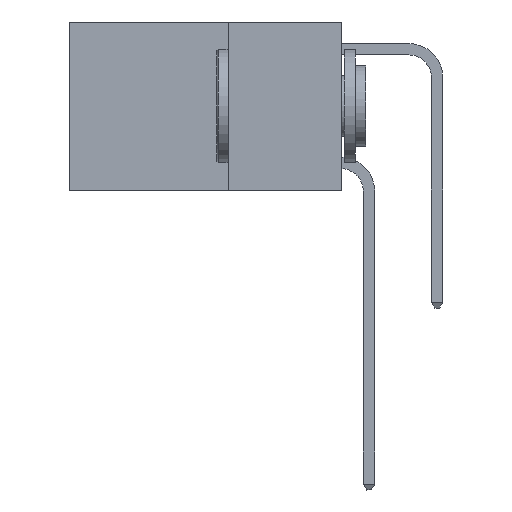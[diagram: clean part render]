
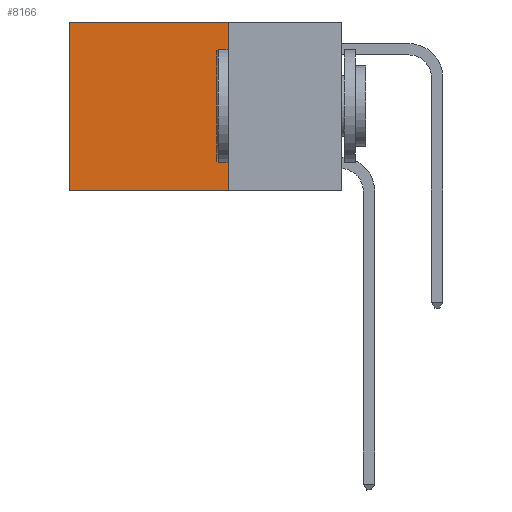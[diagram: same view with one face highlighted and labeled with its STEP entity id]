
A CAD part, left-side view. The second image highlights one B-rep face of the part: STEP entity #8166.
In plain terms, the highlighted planar face has unit normal (-1, 0, 0).
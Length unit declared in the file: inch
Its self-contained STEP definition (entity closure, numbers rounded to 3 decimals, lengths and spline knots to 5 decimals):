
#80 = DIRECTION ( 'NONE',  ( 0., 1., 0. ) ) ;
#1085 = EDGE_LOOP ( 'NONE', ( #6655, #19359, #17851, #24489 ) ) ;
#2685 = VECTOR ( 'NONE', #21482, 39.37008 ) ;
#3974 = PLANE ( 'NONE',  #22488 ) ;
#4721 = VERTEX_POINT ( 'NONE', #11643 ) ;
#5507 = EDGE_CURVE ( 'NONE', #21379, #28579, #24906, .T. ) ;
#6348 = DIRECTION ( 'NONE',  ( 1., 0., 0. ) ) ;
#6655 = ORIENTED_EDGE ( 'NONE', *, *, #5507, .T. ) ;
#7208 = CARTESIAN_POINT ( 'NONE',  ( 0.2625, 0.25, 0. ) ) ;
#8166 = ADVANCED_FACE ( 'NONE', ( #18523 ), #3974, .F. ) ;
#10204 = CARTESIAN_POINT ( 'NONE',  ( 0.2625, 0.25, -0.37 ) ) ;
#10885 = CARTESIAN_POINT ( 'NONE',  ( 0.2625, 0.25, 0. ) ) ;
#11643 = CARTESIAN_POINT ( 'NONE',  ( 0.2625, 0.25, 0. ) ) ;
#12277 = EDGE_CURVE ( 'NONE', #4721, #23978, #16505, .T. ) ;
#13075 = VECTOR ( 'NONE', #80, 39.37008 ) ;
#14367 = CARTESIAN_POINT ( 'NONE',  ( 0.2625, 0.6, -0.37 ) ) ;
#14780 = DIRECTION ( 'NONE',  ( 0., 0., -1. ) ) ;
#16159 = CARTESIAN_POINT ( 'NONE',  ( 0.2625, 0.25, 0. ) ) ;
#16505 = LINE ( 'NONE', #7208, #27000 ) ;
#17851 = ORIENTED_EDGE ( 'NONE', *, *, #12277, .F. ) ;
#18488 = CARTESIAN_POINT ( 'NONE',  ( 0.2625, 0.25, -0.37 ) ) ;
#18523 = FACE_OUTER_BOUND ( 'NONE', #1085, .T. ) ;
#19099 = LINE ( 'NONE', #16159, #13075 ) ;
#19359 = ORIENTED_EDGE ( 'NONE', *, *, #22447, .F. ) ;
#20257 = CARTESIAN_POINT ( 'NONE',  ( 0.2625, 0.6, 0. ) ) ;
#21379 = VERTEX_POINT ( 'NONE', #20257 ) ;
#21482 = DIRECTION ( 'NONE',  ( 0., 1., 0. ) ) ;
#21636 = LINE ( 'NONE', #10204, #2685 ) ;
#22233 = DIRECTION ( 'NONE',  ( 0., 0., -1. ) ) ;
#22447 = EDGE_CURVE ( 'NONE', #23978, #28579, #21636, .T. ) ;
#22488 = AXIS2_PLACEMENT_3D ( 'NONE', #10885, #6348, #22233 ) ;
#23978 = VERTEX_POINT ( 'NONE', #18488 ) ;
#24184 = VECTOR ( 'NONE', #14780, 39.37008 ) ;
#24489 = ORIENTED_EDGE ( 'NONE', *, *, #24702, .T. ) ;
#24702 = EDGE_CURVE ( 'NONE', #4721, #21379, #19099, .T. ) ;
#24906 = LINE ( 'NONE', #25928, #24184 ) ;
#25928 = CARTESIAN_POINT ( 'NONE',  ( 0.2625, 0.6, 0. ) ) ;
#27000 = VECTOR ( 'NONE', #27446, 39.37008 ) ;
#27446 = DIRECTION ( 'NONE',  ( 0., 0., -1. ) ) ;
#28579 = VERTEX_POINT ( 'NONE', #14367 ) ;
